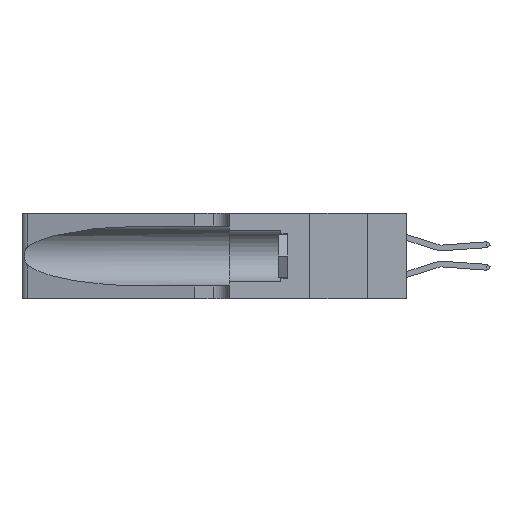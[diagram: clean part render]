
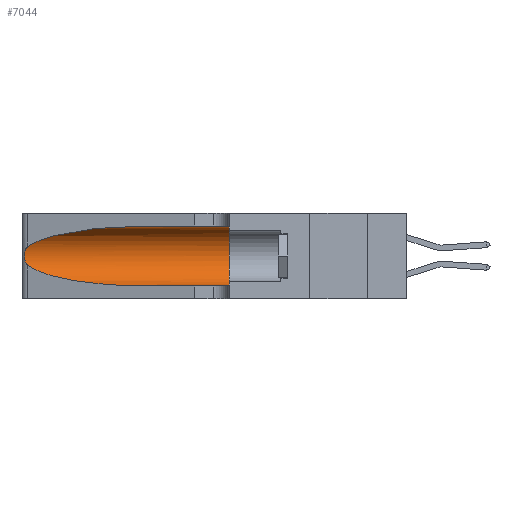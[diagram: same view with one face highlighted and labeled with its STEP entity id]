
A CAD part, left-side view. The second image highlights one B-rep face of the part: STEP entity #7044.
In plain terms, the highlighted cylindrical face has radius 3.308 mm (diameter 6.617 mm), a partial arc.
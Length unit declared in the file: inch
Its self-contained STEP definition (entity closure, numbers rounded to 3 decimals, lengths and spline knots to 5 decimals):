
#347 = CARTESIAN_POINT ( 'NONE',  ( 0.25787, 1.23484, 0.2124 ) ) ;
#974 = CARTESIAN_POINT ( 'NONE',  ( 0.18966, 0.96281, 0.31525 ) ) ;
#998 = VERTEX_POINT ( 'NONE', #23003 ) ;
#1126 = DIRECTION ( 'NONE',  ( 0., -1., 0. ) ) ;
#1158 = EDGE_CURVE ( 'NONE', #14371, #998, #3320, .T. ) ;
#1198 = EDGE_CURVE ( 'NONE', #998, #20958, #3442, .T. ) ;
#1296 = CARTESIAN_POINT ( 'NONE',  ( 0.1305, 0.35, 0.185 ) ) ;
#1587 = EDGE_CURVE ( 'NONE', #21946, #20958, #4306, .T. ) ;
#1947 = CARTESIAN_POINT ( 'NONE',  ( 0.25487, 1.22718, 0.14631 ) ) ;
#2325 = VERTEX_POINT ( 'NONE', #4227 ) ;
#2441 = AXIS2_PLACEMENT_3D ( 'NONE', #19553, #17809, #15011 ) ;
#3320 =( BOUNDED_CURVE ( )  B_SPLINE_CURVE ( 3, ( #3476, #7320, #23507, #20231 ),
 .UNSPECIFIED., .F., .F. ) 
 B_SPLINE_CURVE_WITH_KNOTS ( ( 4, 4 ),
 ( 3.44316, 4.71239 ),
 .UNSPECIFIED. ) 
 CURVE ( )  GEOMETRIC_REPRESENTATION_ITEM ( )  RATIONAL_B_SPLINE_CURVE ( ( 1., 0.87, 0.87, 1. ) ) 
 REPRESENTATION_ITEM ( '' )  );
#3442 = LINE ( 'NONE', #11318, #13762 ) ;
#3476 = CARTESIAN_POINT ( 'NONE',  ( 0.25487, 1.22718, 0.14631 ) ) ;
#4007 = VECTOR ( 'NONE', #1126, 39.37008 ) ;
#4022 = B_SPLINE_CURVE_WITH_KNOTS ( 'NONE', 3,
 ( #20132, #16802, #21897, #347, #12916, #20379, #13003, #10985, #11138, #9205, #5784, #14632, #11062, #1947 ),
 .UNSPECIFIED., .F., .F.,
 ( 4, 2, 2, 2, 2, 2, 4 ),
 ( 0., 0.00027, 0.00053, 0.00107, 0.0016, 0.00187, 0.00214 ),
 .UNSPECIFIED. ) ;
#4115 = DIRECTION ( 'NONE',  ( 0., -1., 0. ) ) ;
#4227 = CARTESIAN_POINT ( 'NONE',  ( 0.25487, 1.22718, 0.22369 ) ) ;
#4306 = CIRCLE ( 'NONE', #8304, 0.13025 ) ;
#5524 = CARTESIAN_POINT ( 'NONE',  ( 0.1305, 0.35, 0.05475 ) ) ;
#5784 = CARTESIAN_POINT ( 'NONE',  ( 0.25789, 1.23486, 0.15765 ) ) ;
#6720 = EDGE_LOOP ( 'NONE', ( #19554, #12645, #9480, #7065, #8234, #14753 ) ) ;
#7044 = ADVANCED_FACE ( 'NONE', ( #21843 ), #7872, .F. ) ;
#7065 = ORIENTED_EDGE ( 'NONE', *, *, #1198, .T. ) ;
#7320 = CARTESIAN_POINT ( 'NONE',  ( 0.2373, 1.15595, 0.08982 ) ) ;
#7872 = CYLINDRICAL_SURFACE ( 'NONE', #2441, 0.13025 ) ;
#8234 = ORIENTED_EDGE ( 'NONE', *, *, #1587, .F. ) ;
#8304 = AXIS2_PLACEMENT_3D ( 'NONE', #1296, #16157, #17916 ) ;
#8405 = CARTESIAN_POINT ( 'NONE',  ( 0.25487, 1.22718, 0.22369 ) ) ;
#9205 = CARTESIAN_POINT ( 'NONE',  ( 0.25856, 1.23593, 0.16098 ) ) ;
#9480 = ORIENTED_EDGE ( 'NONE', *, *, #1158, .T. ) ;
#9931 = CARTESIAN_POINT ( 'NONE',  ( 0.2373, 1.15595, 0.28018 ) ) ;
#10985 = CARTESIAN_POINT ( 'NONE',  ( 0.26075, 1.23896, 0.178 ) ) ;
#11062 = CARTESIAN_POINT ( 'NONE',  ( 0.25555, 1.22993, 0.14849 ) ) ;
#11138 = CARTESIAN_POINT ( 'NONE',  ( 0.26017, 1.23833, 0.17102 ) ) ;
#11318 = CARTESIAN_POINT ( 'NONE',  ( 0.1305, 1.61858, 0.05475 ) ) ;
#11374 =( BOUNDED_CURVE ( )  B_SPLINE_CURVE ( 3, ( #11952, #974, #9931, #8405 ),
 .UNSPECIFIED., .F., .F. ) 
 B_SPLINE_CURVE_WITH_KNOTS ( ( 4, 4 ),
 ( 1.5708, 2.84003 ),
 .UNSPECIFIED. ) 
 CURVE ( )  GEOMETRIC_REPRESENTATION_ITEM ( )  RATIONAL_B_SPLINE_CURVE ( ( 1., 0.87, 0.87, 1. ) ) 
 REPRESENTATION_ITEM ( '' )  );
#11952 = CARTESIAN_POINT ( 'NONE',  ( 0.1305, 0.72297, 0.31525 ) ) ;
#12645 = ORIENTED_EDGE ( 'NONE', *, *, #17518, .T. ) ;
#12916 = CARTESIAN_POINT ( 'NONE',  ( 0.25854, 1.2359, 0.20912 ) ) ;
#13003 = CARTESIAN_POINT ( 'NONE',  ( 0.26075, 1.23896, 0.19203 ) ) ;
#13762 = VECTOR ( 'NONE', #4115, 39.37008 ) ;
#13991 = CARTESIAN_POINT ( 'NONE',  ( 0.1305, 1.61858, 0.31525 ) ) ;
#14353 = EDGE_CURVE ( 'NONE', #17995, #21946, #20290, .T. ) ;
#14371 = VERTEX_POINT ( 'NONE', #23163 ) ;
#14632 = CARTESIAN_POINT ( 'NONE',  ( 0.25639, 1.23186, 0.15144 ) ) ;
#14753 = ORIENTED_EDGE ( 'NONE', *, *, #14353, .F. ) ;
#15011 = DIRECTION ( 'NONE',  ( 0., 0., -1. ) ) ;
#16157 = DIRECTION ( 'NONE',  ( 0., 1., 0. ) ) ;
#16802 = CARTESIAN_POINT ( 'NONE',  ( 0.25555, 1.22994, 0.2215 ) ) ;
#17518 = EDGE_CURVE ( 'NONE', #2325, #14371, #4022, .T. ) ;
#17809 = DIRECTION ( 'NONE',  ( 0., -1., 0. ) ) ;
#17916 = DIRECTION ( 'NONE',  ( 0., 0., 1. ) ) ;
#17995 = VERTEX_POINT ( 'NONE', #23238 ) ;
#19553 = CARTESIAN_POINT ( 'NONE',  ( 0.1305, 1.61858, 0.185 ) ) ;
#19554 = ORIENTED_EDGE ( 'NONE', *, *, #19766, .T. ) ;
#19766 = EDGE_CURVE ( 'NONE', #17995, #2325, #11374, .T. ) ;
#20132 = CARTESIAN_POINT ( 'NONE',  ( 0.25487, 1.22718, 0.22369 ) ) ;
#20231 = CARTESIAN_POINT ( 'NONE',  ( 0.1305, 0.72297, 0.05475 ) ) ;
#20290 = LINE ( 'NONE', #13991, #4007 ) ;
#20379 = CARTESIAN_POINT ( 'NONE',  ( 0.26018, 1.23835, 0.19895 ) ) ;
#20958 = VERTEX_POINT ( 'NONE', #5524 ) ;
#21843 = FACE_OUTER_BOUND ( 'NONE', #6720, .T. ) ;
#21897 = CARTESIAN_POINT ( 'NONE',  ( 0.25639, 1.23184, 0.21858 ) ) ;
#21946 = VERTEX_POINT ( 'NONE', #23276 ) ;
#23003 = CARTESIAN_POINT ( 'NONE',  ( 0.1305, 0.72297, 0.05475 ) ) ;
#23163 = CARTESIAN_POINT ( 'NONE',  ( 0.25487, 1.22718, 0.14631 ) ) ;
#23238 = CARTESIAN_POINT ( 'NONE',  ( 0.1305, 0.72297, 0.31525 ) ) ;
#23276 = CARTESIAN_POINT ( 'NONE',  ( 0.1305, 0.35, 0.31525 ) ) ;
#23507 = CARTESIAN_POINT ( 'NONE',  ( 0.18966, 0.96281, 0.05475 ) ) ;
